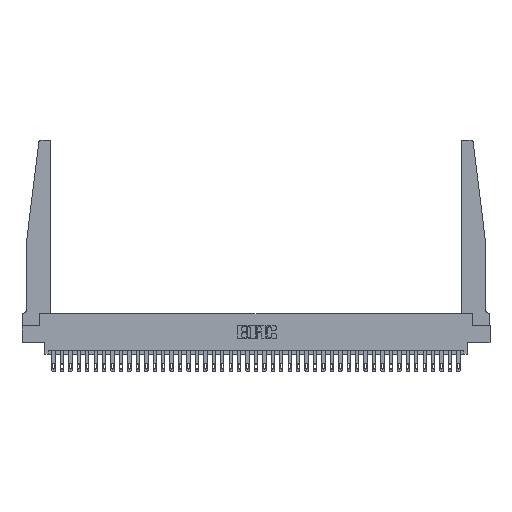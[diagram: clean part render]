
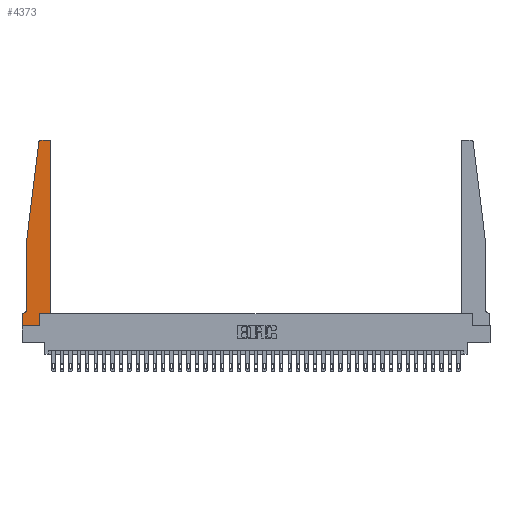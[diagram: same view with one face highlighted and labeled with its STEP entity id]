
A CAD part, top view. The second image highlights one B-rep face of the part: STEP entity #4373.
In plain terms, the highlighted planar face has unit normal (0, 0, 1).
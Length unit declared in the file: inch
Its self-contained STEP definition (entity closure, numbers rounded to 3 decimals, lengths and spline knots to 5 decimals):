
#172 = CARTESIAN_POINT ( 'NONE',  ( 0.425, 0.18, 0.37 ) ) ;
#180 = DIRECTION ( 'NONE',  ( 0., 1., 0. ) ) ;
#648 = DIRECTION ( 'NONE',  ( 0., 0., 1. ) ) ;
#888 = CARTESIAN_POINT ( 'NONE',  ( 0.015, 0.2375, 0.37 ) ) ;
#1183 = CIRCLE ( 'NONE', #35286, 0.03 ) ;
#1932 = AXIS2_PLACEMENT_3D ( 'NONE', #25871, #648, #12211 ) ;
#2171 = CARTESIAN_POINT ( 'NONE',  ( 0., 0.1875, 0.37 ) ) ;
#2734 = LINE ( 'NONE', #172, #25816 ) ;
#2825 = EDGE_CURVE ( 'NONE', #30199, #35402, #5049, .T. ) ;
#2926 = CARTESIAN_POINT ( 'NONE',  ( 0.2605, 0.18, 0.37 ) ) ;
#3003 = CARTESIAN_POINT ( 'NONE',  ( 0.425, 2.72, 0.37 ) ) ;
#3081 = DIRECTION ( 'NONE',  ( 1., 0., 0. ) ) ;
#3140 = CARTESIAN_POINT ( 'NONE',  ( 0., 0., 0.37 ) ) ;
#3372 = CARTESIAN_POINT ( 'NONE',  ( 0.2605, 0., 0.37 ) ) ;
#3610 = LINE ( 'NONE', #17076, #27201 ) ;
#4200 = CARTESIAN_POINT ( 'NONE',  ( 0., 0.1875, 0.37 ) ) ;
#4373 = ADVANCED_FACE ( 'NONE', ( #27405 ), #27039, .T. ) ;
#4889 = CARTESIAN_POINT ( 'NONE',  ( 0.2605, 0.18, 0.37 ) ) ;
#5049 = CIRCLE ( 'NONE', #23876, 0.05 ) ;
#5084 = ORIENTED_EDGE ( 'NONE', *, *, #27641, .T. ) ;
#5179 = DIRECTION ( 'NONE',  ( 0., 0., 1. ) ) ;
#5377 = LINE ( 'NONE', #11627, #19237 ) ;
#6085 = CARTESIAN_POINT ( 'NONE',  ( 0.395, 2.75, 0.37 ) ) ;
#6229 = CARTESIAN_POINT ( 'NONE',  ( 0.065, 0.2375, 0.37 ) ) ;
#8095 = DIRECTION ( 'NONE',  ( -1., 0., 0. ) ) ;
#8678 = VERTEX_POINT ( 'NONE', #12674 ) ;
#9084 = DIRECTION ( 'NONE',  ( 0., -1., 0. ) ) ;
#9521 = DIRECTION ( 'NONE',  ( -1., 0., 0. ) ) ;
#11627 = CARTESIAN_POINT ( 'NONE',  ( 0.25, 2.75, 0.37 ) ) ;
#11904 = CIRCLE ( 'NONE', #1932, 0.03 ) ;
#12211 = DIRECTION ( 'NONE',  ( 1., 0., 0. ) ) ;
#12320 = VERTEX_POINT ( 'NONE', #4200 ) ;
#12525 = ORIENTED_EDGE ( 'NONE', *, *, #2825, .T. ) ;
#12674 = CARTESIAN_POINT ( 'NONE',  ( 0.425, 0.18, 0.37 ) ) ;
#12896 = CARTESIAN_POINT ( 'NONE',  ( 0.425, 0.18, 0.37 ) ) ;
#13194 = ORIENTED_EDGE ( 'NONE', *, *, #16815, .T. ) ;
#13237 = VECTOR ( 'NONE', #9084, 39.37008 ) ;
#13513 = CARTESIAN_POINT ( 'NONE',  ( 0.015, 0.1875, 0.37 ) ) ;
#13976 = CARTESIAN_POINT ( 'NONE',  ( 0.24675, 2.72367, 0.37 ) ) ;
#14089 = VECTOR ( 'NONE', #180, 39.37008 ) ;
#14254 = LINE ( 'NONE', #22731, #13237 ) ;
#14288 = VERTEX_POINT ( 'NONE', #25878 ) ;
#14361 = DIRECTION ( 'NONE',  ( 0., -1., 0. ) ) ;
#15017 = EDGE_CURVE ( 'NONE', #15417, #8678, #2734, .T. ) ;
#15417 = VERTEX_POINT ( 'NONE', #4889 ) ;
#16653 = ORIENTED_EDGE ( 'NONE', *, *, #27578, .T. ) ;
#16789 = VECTOR ( 'NONE', #8095, 39.37008 ) ;
#16815 = EDGE_CURVE ( 'NONE', #33126, #21143, #1183, .T. ) ;
#17076 = CARTESIAN_POINT ( 'NONE',  ( 0., 0., 0.37 ) ) ;
#17368 = VECTOR ( 'NONE', #32803, 39.37008 ) ;
#17793 = VERTEX_POINT ( 'NONE', #3372 ) ;
#17975 = EDGE_CURVE ( 'NONE', #12320, #14288, #19168, .T. ) ;
#18234 = EDGE_LOOP ( 'NONE', ( #33128, #13194, #5084, #20404, #12525, #30670, #28802, #29177, #29237, #20177, #16653, #30982 ) ) ;
#18592 = EDGE_CURVE ( 'NONE', #17793, #15417, #28163, .T. ) ;
#18893 = AXIS2_PLACEMENT_3D ( 'NONE', #2171, #33093, #32746 ) ;
#19168 = LINE ( 'NONE', #3140, #34643 ) ;
#19237 = VECTOR ( 'NONE', #33723, 39.37008 ) ;
#19478 = VERTEX_POINT ( 'NONE', #6085 ) ;
#20177 = ORIENTED_EDGE ( 'NONE', *, *, #15017, .T. ) ;
#20404 = ORIENTED_EDGE ( 'NONE', *, *, #26891, .T. ) ;
#21143 = VERTEX_POINT ( 'NONE', #13976 ) ;
#21755 = EDGE_CURVE ( 'NONE', #14288, #17793, #3610, .T. ) ;
#21868 = DIRECTION ( 'NONE',  ( 1., 0., 0. ) ) ;
#22299 = EDGE_CURVE ( 'NONE', #24051, #19478, #11904, .T. ) ;
#22731 = CARTESIAN_POINT ( 'NONE',  ( 0.065, 1.25, 0.37 ) ) ;
#23876 = AXIS2_PLACEMENT_3D ( 'NONE', #888, #34750, #9521 ) ;
#23919 = CARTESIAN_POINT ( 'NONE',  ( 0.065, 1.25, 0.37 ) ) ;
#24051 = VERTEX_POINT ( 'NONE', #3003 ) ;
#24313 = CARTESIAN_POINT ( 'NONE',  ( 0.065, 1.25, 0.37 ) ) ;
#24699 = LINE ( 'NONE', #12896, #36183 ) ;
#24873 = DIRECTION ( 'NONE',  ( 0., 1., 0. ) ) ;
#25023 = CARTESIAN_POINT ( 'NONE',  ( 0.27653, 2.75, 0.37 ) ) ;
#25054 = LINE ( 'NONE', #33336, #16789 ) ;
#25425 = DIRECTION ( 'NONE',  ( 1., 0., 0. ) ) ;
#25816 = VECTOR ( 'NONE', #21868, 39.37008 ) ;
#25871 = CARTESIAN_POINT ( 'NONE',  ( 0.395, 2.72, 0.37 ) ) ;
#25878 = CARTESIAN_POINT ( 'NONE',  ( 0., 0., 0.37 ) ) ;
#26891 = EDGE_CURVE ( 'NONE', #27997, #30199, #14254, .T. ) ;
#27039 = PLANE ( 'NONE',  #18893 ) ;
#27201 = VECTOR ( 'NONE', #3081, 39.37008 ) ;
#27405 = FACE_OUTER_BOUND ( 'NONE', #18234, .T. ) ;
#27578 = EDGE_CURVE ( 'NONE', #8678, #24051, #24699, .T. ) ;
#27641 = EDGE_CURVE ( 'NONE', #21143, #27997, #35538, .T. ) ;
#27715 = EDGE_CURVE ( 'NONE', #35402, #12320, #25054, .T. ) ;
#27997 = VERTEX_POINT ( 'NONE', #23919 ) ;
#28163 = LINE ( 'NONE', #2926, #14089 ) ;
#28802 = ORIENTED_EDGE ( 'NONE', *, *, #17975, .T. ) ;
#29177 = ORIENTED_EDGE ( 'NONE', *, *, #21755, .T. ) ;
#29237 = ORIENTED_EDGE ( 'NONE', *, *, #18592, .T. ) ;
#30199 = VERTEX_POINT ( 'NONE', #6229 ) ;
#30670 = ORIENTED_EDGE ( 'NONE', *, *, #27715, .T. ) ;
#30777 = CARTESIAN_POINT ( 'NONE',  ( 0.27653, 2.72, 0.37 ) ) ;
#30982 = ORIENTED_EDGE ( 'NONE', *, *, #22299, .T. ) ;
#31412 = EDGE_CURVE ( 'NONE', #19478, #33126, #5377, .T. ) ;
#32746 = DIRECTION ( 'NONE',  ( 1., 0., 0. ) ) ;
#32803 = DIRECTION ( 'NONE',  ( -0.122, -0.992, 0. ) ) ;
#33093 = DIRECTION ( 'NONE',  ( 0., 0., 1. ) ) ;
#33126 = VERTEX_POINT ( 'NONE', #25023 ) ;
#33128 = ORIENTED_EDGE ( 'NONE', *, *, #31412, .T. ) ;
#33336 = CARTESIAN_POINT ( 'NONE',  ( 0.065, 0.1875, 0.37 ) ) ;
#33723 = DIRECTION ( 'NONE',  ( -1., 0., 0. ) ) ;
#34643 = VECTOR ( 'NONE', #14361, 39.37008 ) ;
#34750 = DIRECTION ( 'NONE',  ( 0., 0., -1. ) ) ;
#35286 = AXIS2_PLACEMENT_3D ( 'NONE', #30777, #5179, #25425 ) ;
#35402 = VERTEX_POINT ( 'NONE', #13513 ) ;
#35538 = LINE ( 'NONE', #24313, #17368 ) ;
#36183 = VECTOR ( 'NONE', #24873, 39.37008 ) ;
